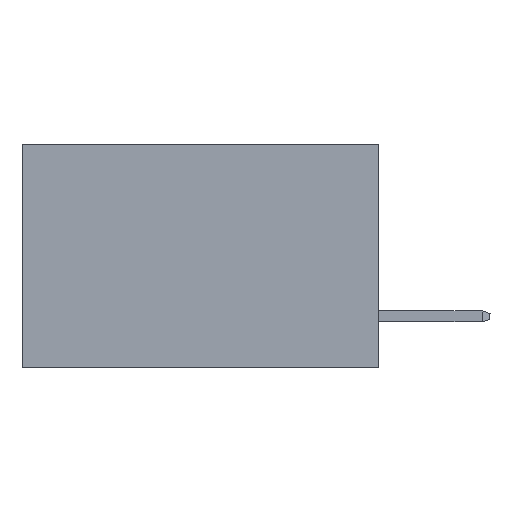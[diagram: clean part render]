
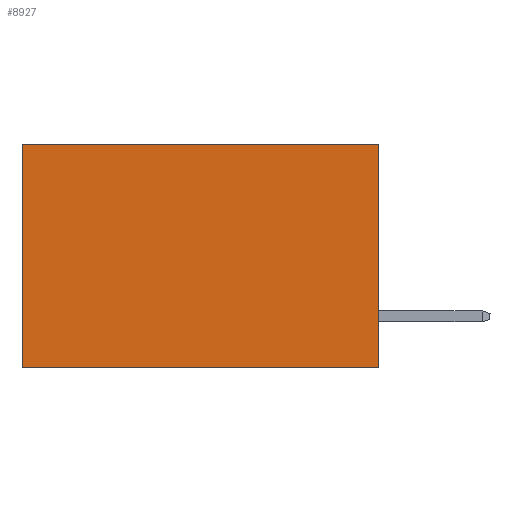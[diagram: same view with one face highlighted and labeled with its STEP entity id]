
A CAD part, left-side view. The second image highlights one B-rep face of the part: STEP entity #8927.
In plain terms, the highlighted planar face has unit normal (-1, 0, 0).
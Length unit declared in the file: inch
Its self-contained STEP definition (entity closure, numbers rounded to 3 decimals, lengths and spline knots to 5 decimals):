
#1121 = CARTESIAN_POINT ( 'NONE',  ( 0.277, 0., 0. ) ) ;
#1312 = EDGE_CURVE ( 'NONE', #8801, #9191, #5089, .T. ) ;
#1361 = DIRECTION ( 'NONE',  ( 0., 0., -1. ) ) ;
#1500 = AXIS2_PLACEMENT_3D ( 'NONE', #6204, #8481, #1361 ) ;
#1956 = DIRECTION ( 'NONE',  ( 0., 0., -1. ) ) ;
#2334 = LINE ( 'NONE', #3029, #10869 ) ;
#3029 = CARTESIAN_POINT ( 'NONE',  ( 0.277, 0., 0. ) ) ;
#3845 = EDGE_CURVE ( 'NONE', #9191, #13284, #11574, .T. ) ;
#4074 = FACE_OUTER_BOUND ( 'NONE', #4342, .T. ) ;
#4216 = DIRECTION ( 'NONE',  ( 0., 1., 0. ) ) ;
#4342 = EDGE_LOOP ( 'NONE', ( #9634, #9548, #8960, #8674 ) ) ;
#5089 = LINE ( 'NONE', #10623, #8113 ) ;
#5871 = VECTOR ( 'NONE', #15043, 39.37008 ) ;
#6153 = PLANE ( 'NONE',  #1500 ) ;
#6204 = CARTESIAN_POINT ( 'NONE',  ( 0.277, 0., -0.37 ) ) ;
#6266 = VECTOR ( 'NONE', #1956, 39.37008 ) ;
#6840 = DIRECTION ( 'NONE',  ( 0., 0., -1. ) ) ;
#8113 = VECTOR ( 'NONE', #6840, 39.37008 ) ;
#8481 = DIRECTION ( 'NONE',  ( 1., 0., 0. ) ) ;
#8674 = ORIENTED_EDGE ( 'NONE', *, *, #14909, .T. ) ;
#8801 = VERTEX_POINT ( 'NONE', #1121 ) ;
#8927 = ADVANCED_FACE ( 'NONE', ( #4074 ), #6153, .F. ) ;
#8960 = ORIENTED_EDGE ( 'NONE', *, *, #1312, .F. ) ;
#8975 = CARTESIAN_POINT ( 'NONE',  ( 0.277, 0.59, -0.37 ) ) ;
#9191 = VERTEX_POINT ( 'NONE', #12204 ) ;
#9342 = EDGE_CURVE ( 'NONE', #10083, #13284, #13927, .T. ) ;
#9548 = ORIENTED_EDGE ( 'NONE', *, *, #3845, .F. ) ;
#9634 = ORIENTED_EDGE ( 'NONE', *, *, #9342, .T. ) ;
#9918 = CARTESIAN_POINT ( 'NONE',  ( 0.277, 0.59, 0. ) ) ;
#10083 = VERTEX_POINT ( 'NONE', #9918 ) ;
#10623 = CARTESIAN_POINT ( 'NONE',  ( 0.277, 0., -0.37 ) ) ;
#10869 = VECTOR ( 'NONE', #4216, 39.37008 ) ;
#11574 = LINE ( 'NONE', #14818, #5871 ) ;
#12204 = CARTESIAN_POINT ( 'NONE',  ( 0.277, 0., -0.37 ) ) ;
#13284 = VERTEX_POINT ( 'NONE', #13474 ) ;
#13474 = CARTESIAN_POINT ( 'NONE',  ( 0.277, 0.59, -0.37 ) ) ;
#13927 = LINE ( 'NONE', #8975, #6266 ) ;
#14818 = CARTESIAN_POINT ( 'NONE',  ( 0.277, 0., -0.37 ) ) ;
#14909 = EDGE_CURVE ( 'NONE', #8801, #10083, #2334, .T. ) ;
#15043 = DIRECTION ( 'NONE',  ( 0., 1., 0. ) ) ;
